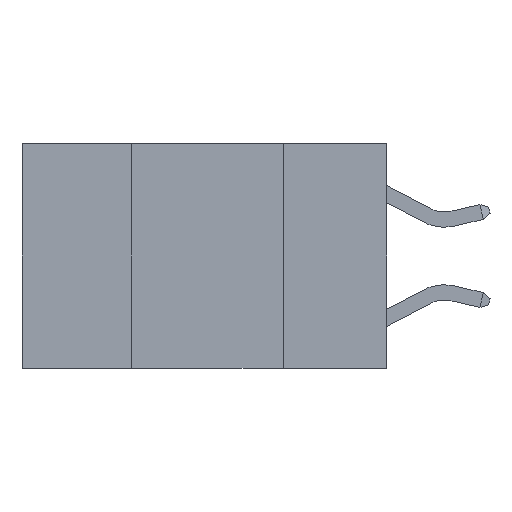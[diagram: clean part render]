
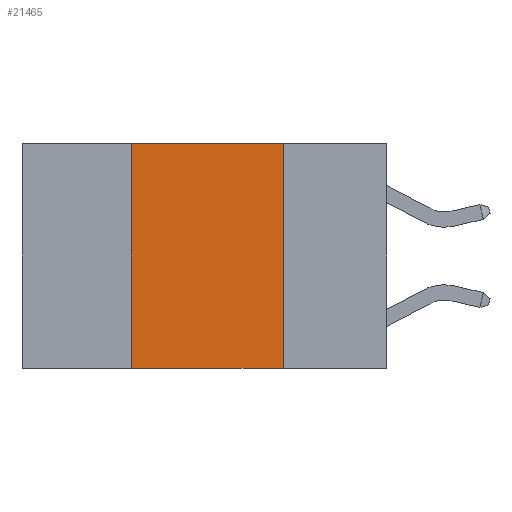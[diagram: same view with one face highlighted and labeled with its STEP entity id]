
A CAD part, left-side view. The second image highlights one B-rep face of the part: STEP entity #21465.
In plain terms, the highlighted planar face has unit normal (-1, 0, 0).
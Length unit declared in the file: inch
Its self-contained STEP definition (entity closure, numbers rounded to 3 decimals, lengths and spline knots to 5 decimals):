
#179 = DIRECTION ( 'NONE',  ( 0., -1., 0. ) ) ;
#1017 = ORIENTED_EDGE ( 'NONE', *, *, #20092, .F. ) ;
#1633 = VERTEX_POINT ( 'NONE', #6352 ) ;
#2320 = DIRECTION ( 'NONE',  ( 0., 0., -1. ) ) ;
#2689 = ORIENTED_EDGE ( 'NONE', *, *, #18954, .F. ) ;
#2945 = VECTOR ( 'NONE', #18630, 39.37008 ) ;
#3058 = CARTESIAN_POINT ( 'NONE',  ( 0., 0.17, -0.37 ) ) ;
#3565 = VERTEX_POINT ( 'NONE', #7778 ) ;
#3922 = ORIENTED_EDGE ( 'NONE', *, *, #6185, .T. ) ;
#5105 = EDGE_CURVE ( 'NONE', #21642, #19173, #6552, .T. ) ;
#5328 = LINE ( 'NONE', #5446, #9594 ) ;
#5382 = LINE ( 'NONE', #20853, #13116 ) ;
#5446 = CARTESIAN_POINT ( 'NONE',  ( 0., 0.6, -0.37 ) ) ;
#6185 = EDGE_CURVE ( 'NONE', #1633, #19173, #5328, .T. ) ;
#6352 = CARTESIAN_POINT ( 'NONE',  ( 0., 0.42, -0.37 ) ) ;
#6552 = LINE ( 'NONE', #16915, #9219 ) ;
#7778 = CARTESIAN_POINT ( 'NONE',  ( 0., 0.42, 0. ) ) ;
#9219 = VECTOR ( 'NONE', #9611, 39.37008 ) ;
#9593 = CARTESIAN_POINT ( 'NONE',  ( 0., 0.17, 0. ) ) ;
#9594 = VECTOR ( 'NONE', #179, 39.37008 ) ;
#9611 = DIRECTION ( 'NONE',  ( 0., 0., -1. ) ) ;
#10635 = PLANE ( 'NONE',  #19169 ) ;
#11877 = CARTESIAN_POINT ( 'NONE',  ( 0., 0.42, 0. ) ) ;
#12909 = FACE_OUTER_BOUND ( 'NONE', #21600, .T. ) ;
#13116 = VECTOR ( 'NONE', #16188, 39.37008 ) ;
#14288 = DIRECTION ( 'NONE',  ( 1., 0., 0. ) ) ;
#16188 = DIRECTION ( 'NONE',  ( 0., -1., 0. ) ) ;
#16915 = CARTESIAN_POINT ( 'NONE',  ( 0., 0.17, 0. ) ) ;
#17937 = CARTESIAN_POINT ( 'NONE',  ( 0., 0.6, 0. ) ) ;
#18630 = DIRECTION ( 'NONE',  ( 0., 0., 1. ) ) ;
#18954 = EDGE_CURVE ( 'NONE', #3565, #21642, #5382, .T. ) ;
#19169 = AXIS2_PLACEMENT_3D ( 'NONE', #17937, #14288, #2320 ) ;
#19173 = VERTEX_POINT ( 'NONE', #3058 ) ;
#20092 = EDGE_CURVE ( 'NONE', #1633, #3565, #20216, .T. ) ;
#20216 = LINE ( 'NONE', #11877, #2945 ) ;
#20853 = CARTESIAN_POINT ( 'NONE',  ( 0., 0.6, 0. ) ) ;
#21399 = ORIENTED_EDGE ( 'NONE', *, *, #5105, .F. ) ;
#21465 = ADVANCED_FACE ( 'NONE', ( #12909 ), #10635, .F. ) ;
#21600 = EDGE_LOOP ( 'NONE', ( #21399, #2689, #1017, #3922 ) ) ;
#21642 = VERTEX_POINT ( 'NONE', #9593 ) ;
